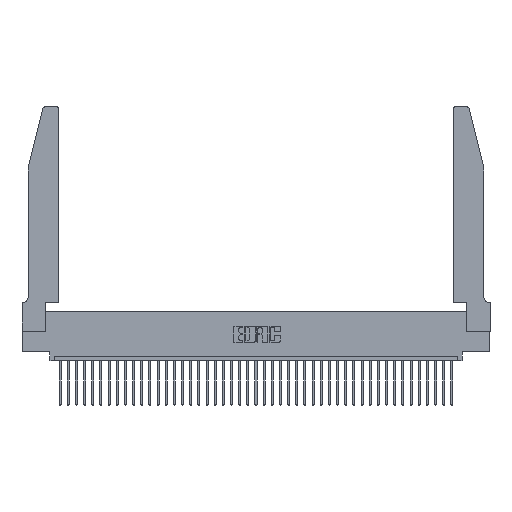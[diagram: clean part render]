
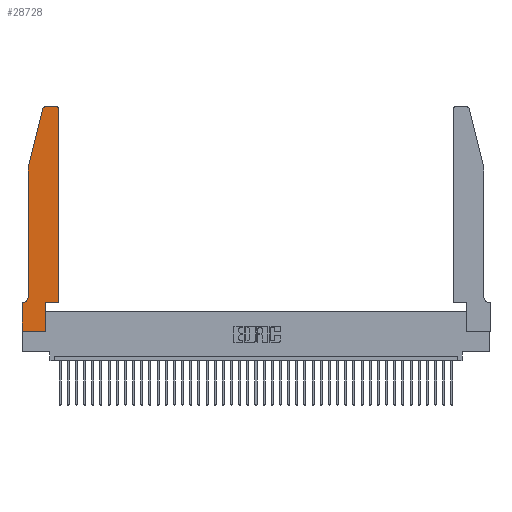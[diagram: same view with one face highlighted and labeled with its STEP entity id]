
A CAD part, top view. The second image highlights one B-rep face of the part: STEP entity #28728.
In plain terms, the highlighted planar face has unit normal (0, 0, 1).
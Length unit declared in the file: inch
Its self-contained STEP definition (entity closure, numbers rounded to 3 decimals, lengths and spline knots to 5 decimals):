
#78 = EDGE_CURVE ( 'NONE', #13314, #18819, #5638, .T. ) ;
#569 = ORIENTED_EDGE ( 'NONE', *, *, #9360, .T. ) ;
#580 = CARTESIAN_POINT ( 'NONE',  ( 0.4205, 2.72, 0.37 ) ) ;
#598 = DIRECTION ( 'NONE',  ( 1., 0., 0. ) ) ;
#1482 = VERTEX_POINT ( 'NONE', #29955 ) ;
#2224 = VERTEX_POINT ( 'NONE', #11397 ) ;
#3477 = VECTOR ( 'NONE', #32481, 39.37008 ) ;
#3620 = LINE ( 'NONE', #40535, #32433 ) ;
#3908 = DIRECTION ( 'NONE',  ( 0., 0., 1. ) ) ;
#4170 = AXIS2_PLACEMENT_3D ( 'NONE', #580, #3908, #10092 ) ;
#4507 = VERTEX_POINT ( 'NONE', #20124 ) ;
#5091 = DIRECTION ( 'NONE',  ( 0., -1., 0. ) ) ;
#5638 = LINE ( 'NONE', #38905, #6558 ) ;
#6306 = CIRCLE ( 'NONE', #6555, 0.07 ) ;
#6346 = CARTESIAN_POINT ( 'NONE',  ( 0.4505, 2.72, 0.37 ) ) ;
#6374 = VECTOR ( 'NONE', #17769, 39.37008 ) ;
#6555 = AXIS2_PLACEMENT_3D ( 'NONE', #34947, #26979, #24530 ) ;
#6558 = VECTOR ( 'NONE', #32521, 39.37008 ) ;
#6812 = LINE ( 'NONE', #7404, #15782 ) ;
#7402 = CARTESIAN_POINT ( 'NONE',  ( 0.2865, 0., 0.37 ) ) ;
#7404 = CARTESIAN_POINT ( 'NONE',  ( 0.2605, 2.75, 0.37 ) ) ;
#7416 = AXIS2_PLACEMENT_3D ( 'NONE', #37678, #15661, #40337 ) ;
#7787 = ORIENTED_EDGE ( 'NONE', *, *, #34621, .T. ) ;
#7800 = LINE ( 'NONE', #36305, #9745 ) ;
#8017 = CARTESIAN_POINT ( 'NONE',  ( 0.284, 2.72, 0.37 ) ) ;
#8036 = CARTESIAN_POINT ( 'NONE',  ( 0., 0., 0.37 ) ) ;
#8207 = EDGE_LOOP ( 'NONE', ( #40181, #20406, #32751, #27200, #32065, #24851, #15444, #569, #11977, #7787, #15687, #24832 ) ) ;
#9360 = EDGE_CURVE ( 'NONE', #15386, #13314, #34421, .T. ) ;
#9697 = VERTEX_POINT ( 'NONE', #29963 ) ;
#9745 = VECTOR ( 'NONE', #23488, 39.37008 ) ;
#10092 = DIRECTION ( 'NONE',  ( 1., 0., 0. ) ) ;
#10361 = CARTESIAN_POINT ( 'NONE',  ( 0.0755, 2., 0.37 ) ) ;
#10588 = DIRECTION ( 'NONE',  ( 0., 0., 1. ) ) ;
#11336 = DIRECTION ( 'NONE',  ( 1., 0., 0. ) ) ;
#11397 = CARTESIAN_POINT ( 'NONE',  ( 0.0755, 0.42, 0.37 ) ) ;
#11977 = ORIENTED_EDGE ( 'NONE', *, *, #78, .T. ) ;
#13314 = VERTEX_POINT ( 'NONE', #7402 ) ;
#14098 = CIRCLE ( 'NONE', #15787, 0.03 ) ;
#15386 = VERTEX_POINT ( 'NONE', #40589 ) ;
#15444 = ORIENTED_EDGE ( 'NONE', *, *, #36302, .T. ) ;
#15555 = CARTESIAN_POINT ( 'NONE',  ( 0., 0.35, 0.37 ) ) ;
#15661 = DIRECTION ( 'NONE',  ( 0., 0., 1. ) ) ;
#15687 = ORIENTED_EDGE ( 'NONE', *, *, #27064, .T. ) ;
#15782 = VECTOR ( 'NONE', #28696, 39.37008 ) ;
#15787 = AXIS2_PLACEMENT_3D ( 'NONE', #8017, #10588, #598 ) ;
#16487 = CARTESIAN_POINT ( 'NONE',  ( 0.0055, 0.35, 0.37 ) ) ;
#16531 = EDGE_CURVE ( 'NONE', #22576, #34322, #31943, .T. ) ;
#17769 = DIRECTION ( 'NONE',  ( -1., 0., 0. ) ) ;
#18367 = LINE ( 'NONE', #35391, #3477 ) ;
#18819 = VERTEX_POINT ( 'NONE', #23178 ) ;
#18822 = DIRECTION ( 'NONE',  ( -0.239, -0.971, 0. ) ) ;
#19596 = VECTOR ( 'NONE', #11336, 39.37008 ) ;
#19619 = VECTOR ( 'NONE', #5091, 39.37008 ) ;
#20124 = CARTESIAN_POINT ( 'NONE',  ( 0.0755, 2., 0.37 ) ) ;
#20406 = ORIENTED_EDGE ( 'NONE', *, *, #24230, .T. ) ;
#22571 = LINE ( 'NONE', #33436, #6374 ) ;
#22576 = VERTEX_POINT ( 'NONE', #6346 ) ;
#23178 = CARTESIAN_POINT ( 'NONE',  ( 0.2865, 0.35, 0.37 ) ) ;
#23488 = DIRECTION ( 'NONE',  ( 0., -1., 0. ) ) ;
#24230 = EDGE_CURVE ( 'NONE', #9697, #1482, #14098, .T. ) ;
#24244 = EDGE_CURVE ( 'NONE', #1482, #4507, #40740, .T. ) ;
#24444 = VERTEX_POINT ( 'NONE', #34029 ) ;
#24530 = DIRECTION ( 'NONE',  ( -1., 0., 0. ) ) ;
#24832 = ORIENTED_EDGE ( 'NONE', *, *, #16531, .T. ) ;
#24851 = ORIENTED_EDGE ( 'NONE', *, *, #26859, .T. ) ;
#25512 = VERTEX_POINT ( 'NONE', #15555 ) ;
#26859 = EDGE_CURVE ( 'NONE', #29618, #25512, #22571, .T. ) ;
#26979 = DIRECTION ( 'NONE',  ( 0., 0., -1. ) ) ;
#27064 = EDGE_CURVE ( 'NONE', #24444, #22576, #3620, .T. ) ;
#27200 = ORIENTED_EDGE ( 'NONE', *, *, #27316, .T. ) ;
#27316 = EDGE_CURVE ( 'NONE', #4507, #2224, #37459, .T. ) ;
#27672 = EDGE_CURVE ( 'NONE', #2224, #29618, #6306, .T. ) ;
#28139 = EDGE_CURVE ( 'NONE', #34322, #9697, #6812, .T. ) ;
#28696 = DIRECTION ( 'NONE',  ( -1., 0., 0. ) ) ;
#28728 = ADVANCED_FACE ( 'NONE', ( #39374 ), #37802, .T. ) ;
#29618 = VERTEX_POINT ( 'NONE', #16487 ) ;
#29955 = CARTESIAN_POINT ( 'NONE',  ( 0.25487, 2.72718, 0.37 ) ) ;
#29963 = CARTESIAN_POINT ( 'NONE',  ( 0.284, 2.75, 0.37 ) ) ;
#30549 = CARTESIAN_POINT ( 'NONE',  ( 0.4205, 2.75, 0.37 ) ) ;
#31943 = CIRCLE ( 'NONE', #4170, 0.03 ) ;
#32065 = ORIENTED_EDGE ( 'NONE', *, *, #27672, .T. ) ;
#32433 = VECTOR ( 'NONE', #37057, 39.37008 ) ;
#32481 = DIRECTION ( 'NONE',  ( 1., 0., 0. ) ) ;
#32521 = DIRECTION ( 'NONE',  ( 0., 1., 0. ) ) ;
#32751 = ORIENTED_EDGE ( 'NONE', *, *, #24244, .T. ) ;
#32763 = VECTOR ( 'NONE', #18822, 39.37008 ) ;
#33436 = CARTESIAN_POINT ( 'NONE',  ( 0.0755, 0.35, 0.37 ) ) ;
#34029 = CARTESIAN_POINT ( 'NONE',  ( 0.4505, 0.35, 0.37 ) ) ;
#34322 = VERTEX_POINT ( 'NONE', #30549 ) ;
#34421 = LINE ( 'NONE', #8036, #19596 ) ;
#34621 = EDGE_CURVE ( 'NONE', #18819, #24444, #18367, .T. ) ;
#34947 = CARTESIAN_POINT ( 'NONE',  ( 0.0055, 0.42, 0.37 ) ) ;
#35391 = CARTESIAN_POINT ( 'NONE',  ( 0.4505, 0.35, 0.37 ) ) ;
#36302 = EDGE_CURVE ( 'NONE', #25512, #15386, #7800, .T. ) ;
#36305 = CARTESIAN_POINT ( 'NONE',  ( 0., 0., 0.37 ) ) ;
#37057 = DIRECTION ( 'NONE',  ( 0., 1., 0. ) ) ;
#37459 = LINE ( 'NONE', #38662, #19619 ) ;
#37678 = CARTESIAN_POINT ( 'NONE',  ( 0., 0.35, 0.37 ) ) ;
#37802 = PLANE ( 'NONE',  #7416 ) ;
#38662 = CARTESIAN_POINT ( 'NONE',  ( 0.0755, 2., 0.37 ) ) ;
#38905 = CARTESIAN_POINT ( 'NONE',  ( 0.2865, 0.35, 0.37 ) ) ;
#39374 = FACE_OUTER_BOUND ( 'NONE', #8207, .T. ) ;
#40181 = ORIENTED_EDGE ( 'NONE', *, *, #28139, .T. ) ;
#40337 = DIRECTION ( 'NONE',  ( 1., 0., 0. ) ) ;
#40535 = CARTESIAN_POINT ( 'NONE',  ( 0.4505, 0.35, 0.37 ) ) ;
#40589 = CARTESIAN_POINT ( 'NONE',  ( 0., 0., 0.37 ) ) ;
#40740 = LINE ( 'NONE', #10361, #32763 ) ;
